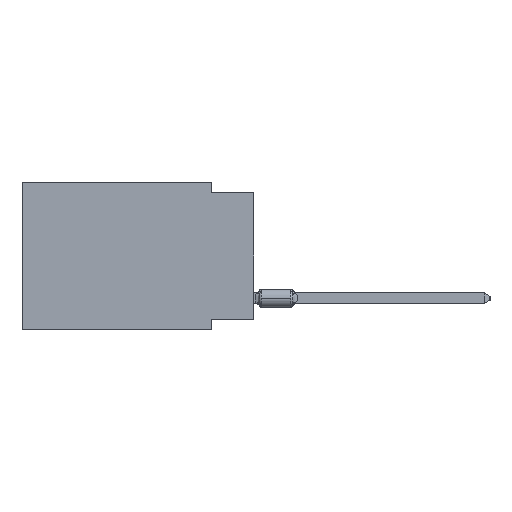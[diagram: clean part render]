
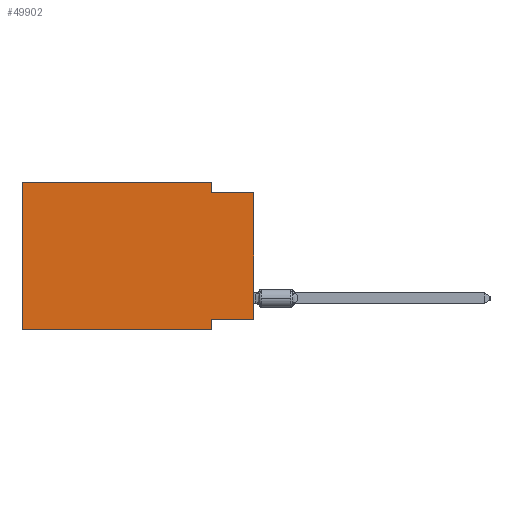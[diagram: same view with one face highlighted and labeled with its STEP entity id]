
A CAD part, left-side view. The second image highlights one B-rep face of the part: STEP entity #49902.
In plain terms, the highlighted planar face has unit normal (-1, 0, 0).
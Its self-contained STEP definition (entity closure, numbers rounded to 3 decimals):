
#1003 = EDGE_CURVE ( 'NONE', #40162, #8167, #52406, .T. ) ;
#1210 = LINE ( 'NONE', #27654, #33532 ) ;
#1981 = EDGE_CURVE ( 'NONE', #40162, #45908, #32971, .T. ) ;
#2113 = ORIENTED_EDGE ( 'NONE', *, *, #1981, .F. ) ;
#2142 = EDGE_CURVE ( 'NONE', #25609, #40865, #34432, .T. ) ;
#4981 = FACE_OUTER_BOUND ( 'NONE', #11092, .T. ) ;
#6092 = CARTESIAN_POINT ( 'NONE',  ( 0., 13.97, 0. ) ) ;
#7755 = VERTEX_POINT ( 'NONE', #44125 ) ;
#8167 = VERTEX_POINT ( 'NONE', #10258 ) ;
#8877 = CARTESIAN_POINT ( 'NONE',  ( 0., 2.54, -8.89 ) ) ;
#10258 = CARTESIAN_POINT ( 'NONE',  ( 0., 2.54, -8.89 ) ) ;
#11092 = EDGE_LOOP ( 'NONE', ( #52695, #29576, #48410, #14606, #2113, #50882, #55936, #25462 ) ) ;
#13184 = DIRECTION ( 'NONE',  ( 0., 1., 0. ) ) ;
#14227 = DIRECTION ( 'NONE',  ( 0., 0., -1. ) ) ;
#14606 = ORIENTED_EDGE ( 'NONE', *, *, #23250, .F. ) ;
#18067 = CARTESIAN_POINT ( 'NONE',  ( 0., 13.97, 0. ) ) ;
#18493 = VERTEX_POINT ( 'NONE', #47004 ) ;
#19239 = DIRECTION ( 'NONE',  ( 1., 0., 0. ) ) ;
#22807 = AXIS2_PLACEMENT_3D ( 'NONE', #45651, #19239, #41786 ) ;
#23123 = LINE ( 'NONE', #8877, #44955 ) ;
#23250 = EDGE_CURVE ( 'NONE', #45908, #18493, #45350, .T. ) ;
#23639 = CARTESIAN_POINT ( 'NONE',  ( 0., 0., -0.635 ) ) ;
#23806 = VECTOR ( 'NONE', #13184, 1000. ) ;
#23905 = DIRECTION ( 'NONE',  ( 0., 0., -1. ) ) ;
#24664 = CARTESIAN_POINT ( 'NONE',  ( 0., 0., -0.635 ) ) ;
#25462 = ORIENTED_EDGE ( 'NONE', *, *, #33287, .F. ) ;
#25609 = VERTEX_POINT ( 'NONE', #43434 ) ;
#27654 = CARTESIAN_POINT ( 'NONE',  ( 0., 0., 0. ) ) ;
#27749 = VECTOR ( 'NONE', #36166, 1000. ) ;
#28348 = CARTESIAN_POINT ( 'NONE',  ( 0., 2.54, 0. ) ) ;
#28524 = CARTESIAN_POINT ( 'NONE',  ( 0., 13.97, 0. ) ) ;
#29576 = ORIENTED_EDGE ( 'NONE', *, *, #2142, .F. ) ;
#32971 = LINE ( 'NONE', #28524, #35630 ) ;
#33287 = EDGE_CURVE ( 'NONE', #36371, #7755, #45220, .T. ) ;
#33532 = VECTOR ( 'NONE', #45463, 1000. ) ;
#34432 = LINE ( 'NONE', #24664, #48888 ) ;
#35630 = VECTOR ( 'NONE', #50790, 1000. ) ;
#36166 = DIRECTION ( 'NONE',  ( 0., -1., 0. ) ) ;
#36371 = VERTEX_POINT ( 'NONE', #48156 ) ;
#37588 = EDGE_CURVE ( 'NONE', #18493, #25609, #47061, .T. ) ;
#38298 = DIRECTION ( 'NONE',  ( 0., -1., 0. ) ) ;
#40162 = VERTEX_POINT ( 'NONE', #55017 ) ;
#40247 = VECTOR ( 'NONE', #42623, 1000. ) ;
#40865 = VERTEX_POINT ( 'NONE', #23639 ) ;
#41751 = EDGE_CURVE ( 'NONE', #36371, #40865, #1210, .T. ) ;
#41770 = VECTOR ( 'NONE', #23905, 1000. ) ;
#41786 = DIRECTION ( 'NONE',  ( 0., 0., -1. ) ) ;
#42142 = EDGE_CURVE ( 'NONE', #7755, #8167, #23123, .T. ) ;
#42623 = DIRECTION ( 'NONE',  ( 0., -1., 0. ) ) ;
#43434 = CARTESIAN_POINT ( 'NONE',  ( 0., 2.54, -0.635 ) ) ;
#44125 = CARTESIAN_POINT ( 'NONE',  ( 0., 2.54, -8.255 ) ) ;
#44955 = VECTOR ( 'NONE', #14227, 1000. ) ;
#45220 = LINE ( 'NONE', #53835, #23806 ) ;
#45350 = LINE ( 'NONE', #18067, #27749 ) ;
#45463 = DIRECTION ( 'NONE',  ( 0., 0., 1. ) ) ;
#45651 = CARTESIAN_POINT ( 'NONE',  ( 0., 13.97, 0. ) ) ;
#45908 = VERTEX_POINT ( 'NONE', #6092 ) ;
#47004 = CARTESIAN_POINT ( 'NONE',  ( 0., 2.54, 0. ) ) ;
#47061 = LINE ( 'NONE', #28348, #41770 ) ;
#48156 = CARTESIAN_POINT ( 'NONE',  ( 0., 0., -8.255 ) ) ;
#48410 = ORIENTED_EDGE ( 'NONE', *, *, #37588, .F. ) ;
#48888 = VECTOR ( 'NONE', #38298, 1000. ) ;
#49902 = ADVANCED_FACE ( 'NONE', ( #4981 ), #54553, .F. ) ;
#50790 = DIRECTION ( 'NONE',  ( 0., 0., 1. ) ) ;
#50882 = ORIENTED_EDGE ( 'NONE', *, *, #1003, .T. ) ;
#52120 = CARTESIAN_POINT ( 'NONE',  ( 0., 13.97, -8.89 ) ) ;
#52406 = LINE ( 'NONE', #52120, #40247 ) ;
#52695 = ORIENTED_EDGE ( 'NONE', *, *, #41751, .T. ) ;
#53835 = CARTESIAN_POINT ( 'NONE',  ( 0., 0., -8.255 ) ) ;
#54553 = PLANE ( 'NONE',  #22807 ) ;
#55017 = CARTESIAN_POINT ( 'NONE',  ( 0., 13.97, -8.89 ) ) ;
#55936 = ORIENTED_EDGE ( 'NONE', *, *, #42142, .F. ) ;
